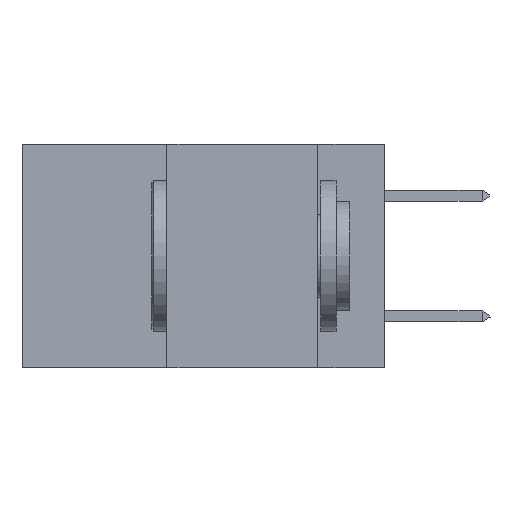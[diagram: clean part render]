
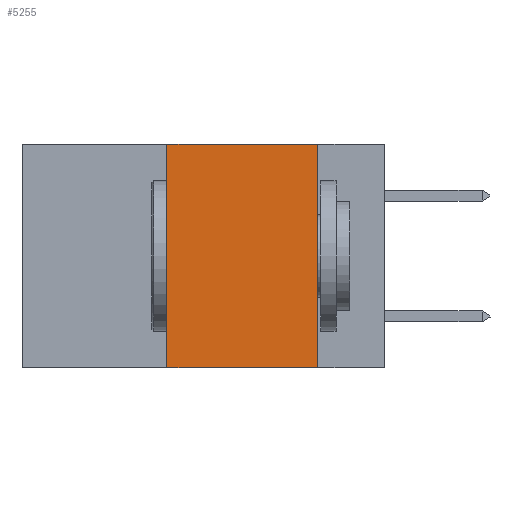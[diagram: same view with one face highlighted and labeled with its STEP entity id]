
A CAD part, left-side view. The second image highlights one B-rep face of the part: STEP entity #5255.
In plain terms, the highlighted planar face has unit normal (-1, 0, 0).
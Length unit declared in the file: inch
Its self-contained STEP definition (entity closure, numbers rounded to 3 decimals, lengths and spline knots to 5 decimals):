
#1560 = CARTESIAN_POINT ( 'NONE',  ( 0., 0.36, 0. ) ) ;
#2609 = DIRECTION ( 'NONE',  ( 1., 0., 0. ) ) ;
#2906 = CARTESIAN_POINT ( 'NONE',  ( 0., 0.11, 0. ) ) ;
#3047 = CARTESIAN_POINT ( 'NONE',  ( 0., 0.11, 0. ) ) ;
#3289 = ORIENTED_EDGE ( 'NONE', *, *, #16825, .F. ) ;
#3414 = LINE ( 'NONE', #39057, #6412 ) ;
#4553 = LINE ( 'NONE', #2906, #11647 ) ;
#5255 = ADVANCED_FACE ( 'NONE', ( #17831 ), #9216, .F. ) ;
#5781 = CARTESIAN_POINT ( 'NONE',  ( 0., 0.6, 0. ) ) ;
#5785 = VECTOR ( 'NONE', #38077, 39.37008 ) ;
#6103 = CARTESIAN_POINT ( 'NONE',  ( 0., 0.6, 0. ) ) ;
#6412 = VECTOR ( 'NONE', #12978, 39.37008 ) ;
#7315 = EDGE_LOOP ( 'NONE', ( #25244, #3289, #15452, #35007 ) ) ;
#7526 = VERTEX_POINT ( 'NONE', #1560 ) ;
#9216 = PLANE ( 'NONE',  #16739 ) ;
#9384 = DIRECTION ( 'NONE',  ( 0., 0., -1. ) ) ;
#11647 = VECTOR ( 'NONE', #9384, 39.37008 ) ;
#12978 = DIRECTION ( 'NONE',  ( 0., 0., 1. ) ) ;
#13320 = VERTEX_POINT ( 'NONE', #3047 ) ;
#15167 = CARTESIAN_POINT ( 'NONE',  ( 0., 0.36, -0.37 ) ) ;
#15452 = ORIENTED_EDGE ( 'NONE', *, *, #28795, .F. ) ;
#16739 = AXIS2_PLACEMENT_3D ( 'NONE', #6103, #2609, #21898 ) ;
#16825 = EDGE_CURVE ( 'NONE', #7526, #13320, #24950, .T. ) ;
#17831 = FACE_OUTER_BOUND ( 'NONE', #7315, .T. ) ;
#18622 = LINE ( 'NONE', #23026, #25171 ) ;
#19056 = EDGE_CURVE ( 'NONE', #13320, #28188, #4553, .T. ) ;
#20350 = EDGE_CURVE ( 'NONE', #33992, #28188, #18622, .T. ) ;
#21898 = DIRECTION ( 'NONE',  ( 0., 0., -1. ) ) ;
#23026 = CARTESIAN_POINT ( 'NONE',  ( 0., 0.6, -0.37 ) ) ;
#24950 = LINE ( 'NONE', #5781, #5785 ) ;
#25171 = VECTOR ( 'NONE', #26295, 39.37008 ) ;
#25244 = ORIENTED_EDGE ( 'NONE', *, *, #19056, .F. ) ;
#26295 = DIRECTION ( 'NONE',  ( 0., -1., 0. ) ) ;
#28188 = VERTEX_POINT ( 'NONE', #39101 ) ;
#28795 = EDGE_CURVE ( 'NONE', #33992, #7526, #3414, .T. ) ;
#33992 = VERTEX_POINT ( 'NONE', #15167 ) ;
#35007 = ORIENTED_EDGE ( 'NONE', *, *, #20350, .T. ) ;
#38077 = DIRECTION ( 'NONE',  ( 0., -1., 0. ) ) ;
#39057 = CARTESIAN_POINT ( 'NONE',  ( 0., 0.36, 0. ) ) ;
#39101 = CARTESIAN_POINT ( 'NONE',  ( 0., 0.11, -0.37 ) ) ;
